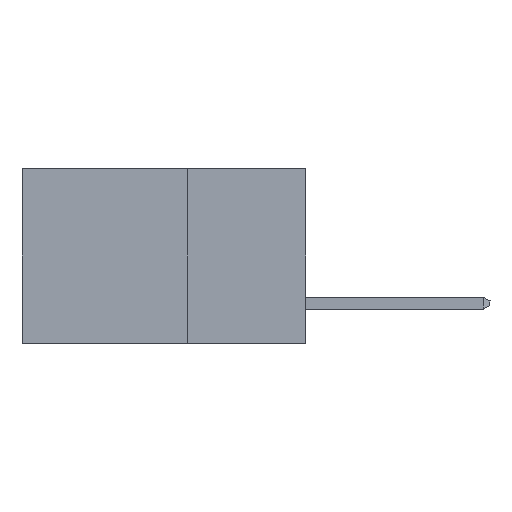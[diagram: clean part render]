
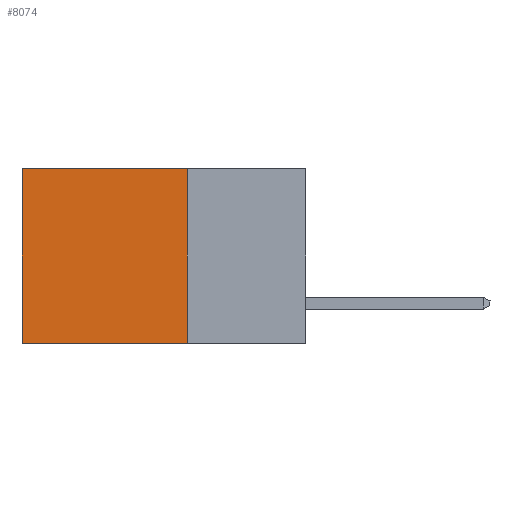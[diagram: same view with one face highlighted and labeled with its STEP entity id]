
A CAD part, left-side view. The second image highlights one B-rep face of the part: STEP entity #8074.
In plain terms, the highlighted planar face has unit normal (-1, 0, 0).
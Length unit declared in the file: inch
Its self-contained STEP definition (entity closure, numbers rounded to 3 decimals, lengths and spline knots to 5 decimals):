
#128 = EDGE_CURVE ( 'NONE', #7211, #5185, #9783, .T. ) ;
#301 = DIRECTION ( 'NONE',  ( 0., 0., -1. ) ) ;
#323 = VECTOR ( 'NONE', #2604, 39.37008 ) ;
#523 = VECTOR ( 'NONE', #5412, 39.37008 ) ;
#668 = CARTESIAN_POINT ( 'NONE',  ( 0.298, 0.25, 0. ) ) ;
#851 = EDGE_LOOP ( 'NONE', ( #6756, #2407, #3644, #8447 ) ) ;
#1764 = CARTESIAN_POINT ( 'NONE',  ( 0.298, 0.25, -0.37 ) ) ;
#2085 = EDGE_CURVE ( 'NONE', #10055, #10703, #7193, .T. ) ;
#2227 = CARTESIAN_POINT ( 'NONE',  ( 0.298, 0.25, -0.37 ) ) ;
#2407 = ORIENTED_EDGE ( 'NONE', *, *, #2085, .F. ) ;
#2604 = DIRECTION ( 'NONE',  ( 0., 1., 0. ) ) ;
#3644 = ORIENTED_EDGE ( 'NONE', *, *, #7166, .F. ) ;
#3696 = CARTESIAN_POINT ( 'NONE',  ( 0.298, 0.6, 0. ) ) ;
#3716 = CARTESIAN_POINT ( 'NONE',  ( 0.298, 0.25, 0. ) ) ;
#5185 = VERTEX_POINT ( 'NONE', #10096 ) ;
#5313 = DIRECTION ( 'NONE',  ( 0., 0., -1. ) ) ;
#5412 = DIRECTION ( 'NONE',  ( 0., 1., 0. ) ) ;
#5421 = LINE ( 'NONE', #9509, #6203 ) ;
#5967 = AXIS2_PLACEMENT_3D ( 'NONE', #9467, #6103, #10365 ) ;
#6103 = DIRECTION ( 'NONE',  ( 1., 0., 0. ) ) ;
#6203 = VECTOR ( 'NONE', #5313, 39.37008 ) ;
#6756 = ORIENTED_EDGE ( 'NONE', *, *, #7389, .T. ) ;
#7166 = EDGE_CURVE ( 'NONE', #7211, #10055, #5421, .T. ) ;
#7193 = LINE ( 'NONE', #1764, #323 ) ;
#7211 = VERTEX_POINT ( 'NONE', #668 ) ;
#7233 = VECTOR ( 'NONE', #301, 39.37008 ) ;
#7389 = EDGE_CURVE ( 'NONE', #5185, #10703, #10033, .T. ) ;
#8074 = ADVANCED_FACE ( 'NONE', ( #8830 ), #9399, .F. ) ;
#8447 = ORIENTED_EDGE ( 'NONE', *, *, #128, .T. ) ;
#8830 = FACE_OUTER_BOUND ( 'NONE', #851, .T. ) ;
#9399 = PLANE ( 'NONE',  #5967 ) ;
#9467 = CARTESIAN_POINT ( 'NONE',  ( 0.298, 0.25, 0. ) ) ;
#9509 = CARTESIAN_POINT ( 'NONE',  ( 0.298, 0.25, 0. ) ) ;
#9783 = LINE ( 'NONE', #3716, #523 ) ;
#10033 = LINE ( 'NONE', #3696, #7233 ) ;
#10055 = VERTEX_POINT ( 'NONE', #2227 ) ;
#10096 = CARTESIAN_POINT ( 'NONE',  ( 0.298, 0.6, 0. ) ) ;
#10365 = DIRECTION ( 'NONE',  ( 0., 0., -1. ) ) ;
#10703 = VERTEX_POINT ( 'NONE', #10977 ) ;
#10977 = CARTESIAN_POINT ( 'NONE',  ( 0.298, 0.6, -0.37 ) ) ;
